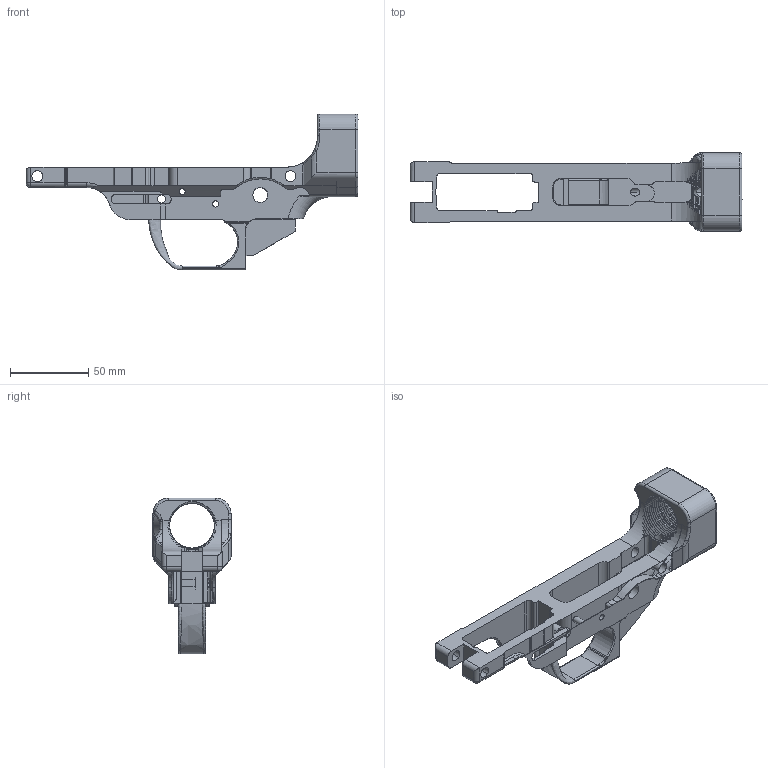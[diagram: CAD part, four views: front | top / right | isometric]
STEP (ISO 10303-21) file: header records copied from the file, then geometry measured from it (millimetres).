
FILE_DESCRIPTION (( 'STEP AP214' ), '1' );
FILE_NAME ('Phobos_V1.2.STEP', '2015-05-21T06:07:43', ( 'WarFairy' ), ( '' ), 'SwSTEP 2.0', 'SolidWorks 2015', '' );
FILE_SCHEMA (( 'AUTOMOTIVE_DESIGN' ));
Length unit declared in the file: inch
Products named in the file (1): Phobos_V1.2
Bounding box: 212.37 x 50 x 99.72 mm (x, y, z)
Volume: 144024.2 mm3; surface area: 49008.2 mm2
Topology: 1 solids, 1 shells, 475 faces, 1373 edges, 880 vertices
Faces by surface type: cylinder 216, plane 122, bspline 82, torus 34, cone 17, sphere 4
Entity records: 33303 total; most frequent: CARTESIAN_POINT 21945, ORIENTED_EDGE 2726, DIRECTION 1920, EDGE_CURVE 1363, VERTEX_POINT 880, AXIS2_PLACEMENT_3D 701, VECTOR 518, LINE 518
